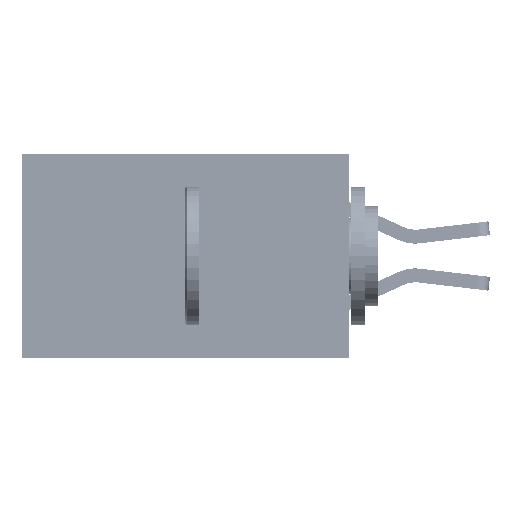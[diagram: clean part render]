
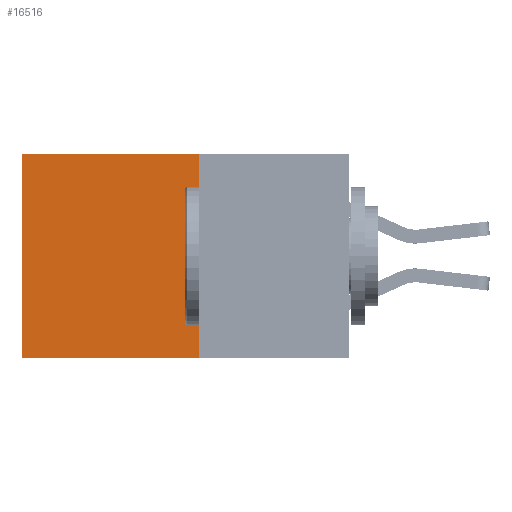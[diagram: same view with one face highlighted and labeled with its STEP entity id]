
A CAD part, left-side view. The second image highlights one B-rep face of the part: STEP entity #16516.
In plain terms, the highlighted planar face has unit normal (-1, 0, 0).
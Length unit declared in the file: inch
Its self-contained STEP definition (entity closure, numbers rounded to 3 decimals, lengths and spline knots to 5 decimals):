
#170 = CARTESIAN_POINT ( 'NONE',  ( 0.277, 0.27, -0.37 ) ) ;
#526 = VERTEX_POINT ( 'NONE', #34013 ) ;
#818 = EDGE_CURVE ( 'NONE', #6800, #8143, #18820, .T. ) ;
#2105 = VECTOR ( 'NONE', #18972, 39.37008 ) ;
#2515 = VERTEX_POINT ( 'NONE', #7571 ) ;
#3395 = LINE ( 'NONE', #25407, #31848 ) ;
#4701 = AXIS2_PLACEMENT_3D ( 'NONE', #29276, #13270, #31907 ) ;
#6800 = VERTEX_POINT ( 'NONE', #31780 ) ;
#7092 = EDGE_CURVE ( 'NONE', #2515, #526, #16215, .T. ) ;
#7571 = CARTESIAN_POINT ( 'NONE',  ( 0.277, 0.27, 0. ) ) ;
#7678 = ORIENTED_EDGE ( 'NONE', *, *, #7092, .F. ) ;
#8143 = VERTEX_POINT ( 'NONE', #23438 ) ;
#8875 = DIRECTION ( 'NONE',  ( 0., 0., -1. ) ) ;
#9362 = CARTESIAN_POINT ( 'NONE',  ( 0.277, 0.59, -0.37 ) ) ;
#9386 = DIRECTION ( 'NONE',  ( 0., 1., 0. ) ) ;
#11194 = ORIENTED_EDGE ( 'NONE', *, *, #13281, .T. ) ;
#11694 = VECTOR ( 'NONE', #31522, 39.37008 ) ;
#13270 = DIRECTION ( 'NONE',  ( 1., 0., 0. ) ) ;
#13281 = EDGE_CURVE ( 'NONE', #2515, #6800, #3395, .T. ) ;
#14304 = EDGE_LOOP ( 'NONE', ( #16461, #27325, #7678, #11194 ) ) ;
#15846 = PLANE ( 'NONE',  #4701 ) ;
#16215 = LINE ( 'NONE', #24916, #22476 ) ;
#16461 = ORIENTED_EDGE ( 'NONE', *, *, #818, .T. ) ;
#16516 = ADVANCED_FACE ( 'NONE', ( #20830 ), #15846, .F. ) ;
#18820 = LINE ( 'NONE', #9362, #11694 ) ;
#18972 = DIRECTION ( 'NONE',  ( 0., 1., 0. ) ) ;
#20830 = FACE_OUTER_BOUND ( 'NONE', #14304, .T. ) ;
#22476 = VECTOR ( 'NONE', #8875, 39.37008 ) ;
#22670 = LINE ( 'NONE', #170, #2105 ) ;
#23438 = CARTESIAN_POINT ( 'NONE',  ( 0.277, 0.59, -0.37 ) ) ;
#24916 = CARTESIAN_POINT ( 'NONE',  ( 0.277, 0.27, -0.37 ) ) ;
#25407 = CARTESIAN_POINT ( 'NONE',  ( 0.277, 0.27, 0. ) ) ;
#27325 = ORIENTED_EDGE ( 'NONE', *, *, #34201, .F. ) ;
#29276 = CARTESIAN_POINT ( 'NONE',  ( 0.277, 0.27, -0.37 ) ) ;
#31522 = DIRECTION ( 'NONE',  ( 0., 0., -1. ) ) ;
#31780 = CARTESIAN_POINT ( 'NONE',  ( 0.277, 0.59, 0. ) ) ;
#31848 = VECTOR ( 'NONE', #9386, 39.37008 ) ;
#31907 = DIRECTION ( 'NONE',  ( 0., 0., -1. ) ) ;
#34013 = CARTESIAN_POINT ( 'NONE',  ( 0.277, 0.27, -0.37 ) ) ;
#34201 = EDGE_CURVE ( 'NONE', #526, #8143, #22670, .T. ) ;
